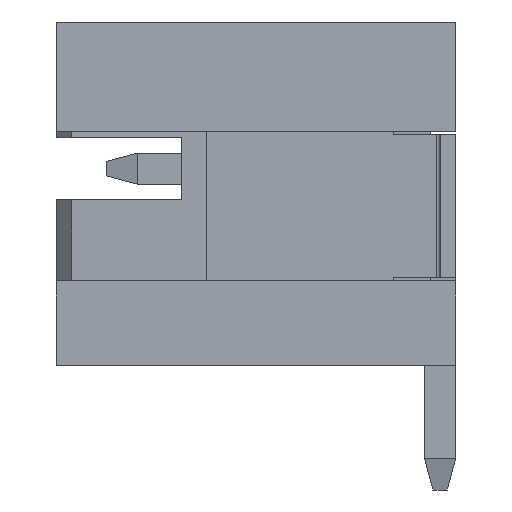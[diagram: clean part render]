
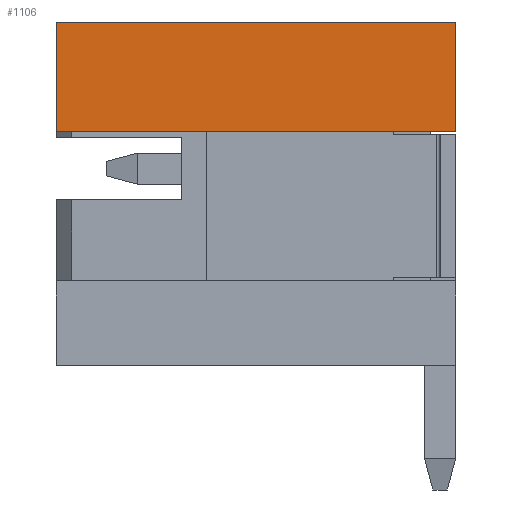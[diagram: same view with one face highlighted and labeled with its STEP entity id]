
A CAD part, left-side view. The second image highlights one B-rep face of the part: STEP entity #1106.
In plain terms, the highlighted planar face has unit normal (-1, 0, 0).
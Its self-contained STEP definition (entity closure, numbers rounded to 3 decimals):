
#68 = PLANE ( 'NONE',  #2617 ) ;
#113 = CARTESIAN_POINT ( 'NONE',  ( -3., 0., 0. ) ) ;
#242 = CARTESIAN_POINT ( 'NONE',  ( -3., 0., 2.35 ) ) ;
#360 = EDGE_LOOP ( 'NONE', ( #3326, #1716, #4341, #4457 ) ) ;
#506 = DIRECTION ( 'NONE',  ( 1., 0., 0. ) ) ;
#923 = EDGE_CURVE ( 'NONE', #4401, #2610, #2194, .T. ) ;
#972 = CARTESIAN_POINT ( 'NONE',  ( -3., 0., 0.6 ) ) ;
#1056 = EDGE_CURVE ( 'NONE', #3518, #4401, #1089, .T. ) ;
#1089 = LINE ( 'NONE', #3881, #2313 ) ;
#1106 = ADVANCED_FACE ( 'NONE', ( #4549 ), #68, .F. ) ;
#1212 = DIRECTION ( 'NONE',  ( 0., 0., -1. ) ) ;
#1224 = VERTEX_POINT ( 'NONE', #3189 ) ;
#1431 = EDGE_CURVE ( 'NONE', #2610, #1224, #2946, .T. ) ;
#1640 = CARTESIAN_POINT ( 'NONE',  ( -3., 6.4, 2.35 ) ) ;
#1716 = ORIENTED_EDGE ( 'NONE', *, *, #1056, .F. ) ;
#2077 = CARTESIAN_POINT ( 'NONE',  ( -3., 6.4, 0.6 ) ) ;
#2152 = CARTESIAN_POINT ( 'NONE',  ( -3., 6.4, 2.35 ) ) ;
#2194 = LINE ( 'NONE', #3776, #4722 ) ;
#2246 = DIRECTION ( 'NONE',  ( 0., 0., 1. ) ) ;
#2313 = VECTOR ( 'NONE', #4209, 1000. ) ;
#2610 = VERTEX_POINT ( 'NONE', #1640 ) ;
#2617 = AXIS2_PLACEMENT_3D ( 'NONE', #113, #506, #1212 ) ;
#2946 = LINE ( 'NONE', #2152, #4835 ) ;
#3189 = CARTESIAN_POINT ( 'NONE',  ( -3., 0., 2.35 ) ) ;
#3241 = DIRECTION ( 'NONE',  ( 0., 0., -1. ) ) ;
#3296 = EDGE_CURVE ( 'NONE', #1224, #3518, #4119, .T. ) ;
#3326 = ORIENTED_EDGE ( 'NONE', *, *, #923, .F. ) ;
#3518 = VERTEX_POINT ( 'NONE', #972 ) ;
#3533 = VECTOR ( 'NONE', #3241, 1000. ) ;
#3776 = CARTESIAN_POINT ( 'NONE',  ( -3., 6.4, 2.35 ) ) ;
#3881 = CARTESIAN_POINT ( 'NONE',  ( -3., 0., 0.6 ) ) ;
#4119 = LINE ( 'NONE', #242, #3533 ) ;
#4209 = DIRECTION ( 'NONE',  ( 0., 1., 0. ) ) ;
#4341 = ORIENTED_EDGE ( 'NONE', *, *, #3296, .F. ) ;
#4401 = VERTEX_POINT ( 'NONE', #2077 ) ;
#4457 = ORIENTED_EDGE ( 'NONE', *, *, #1431, .F. ) ;
#4549 = FACE_OUTER_BOUND ( 'NONE', #360, .T. ) ;
#4722 = VECTOR ( 'NONE', #2246, 1000. ) ;
#4780 = DIRECTION ( 'NONE',  ( 0., -1., 0. ) ) ;
#4835 = VECTOR ( 'NONE', #4780, 1000. ) ;
